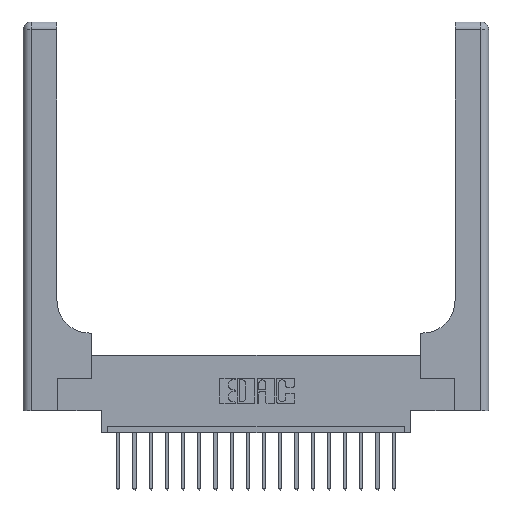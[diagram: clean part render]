
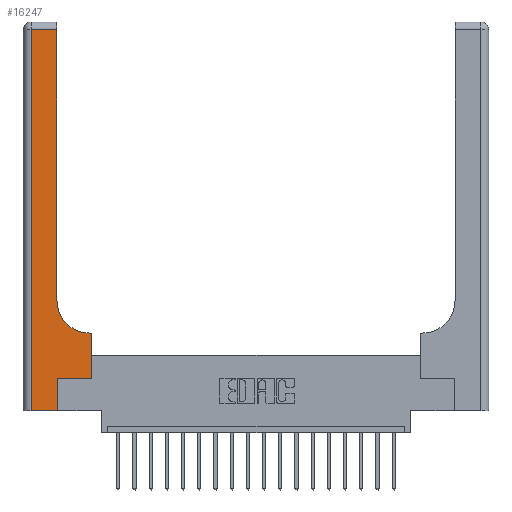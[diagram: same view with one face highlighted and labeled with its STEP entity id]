
A CAD part, top view. The second image highlights one B-rep face of the part: STEP entity #16247.
In plain terms, the highlighted planar face has unit normal (0, 0, 1).
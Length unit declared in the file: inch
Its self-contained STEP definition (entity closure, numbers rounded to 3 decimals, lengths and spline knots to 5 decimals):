
#728 = ORIENTED_EDGE ( 'NONE', *, *, #10570, .T. ) ;
#733 = FACE_OUTER_BOUND ( 'NONE', #19905, .T. ) ;
#1167 = CARTESIAN_POINT ( 'NONE',  ( 0.51, 0.6, 0.37 ) ) ;
#1189 = ORIENTED_EDGE ( 'NONE', *, *, #10052, .T. ) ;
#1239 = ORIENTED_EDGE ( 'NONE', *, *, #1798, .T. ) ;
#1676 = CARTESIAN_POINT ( 'NONE',  ( 0.51, 0.85, 0.37 ) ) ;
#1798 = EDGE_CURVE ( 'NONE', #15575, #12242, #14956, .T. ) ;
#2239 = CARTESIAN_POINT ( 'NONE',  ( 0.06, 0., 0.37 ) ) ;
#2600 = CARTESIAN_POINT ( 'NONE',  ( 0.26, 0.6, 0.37 ) ) ;
#2780 = ORIENTED_EDGE ( 'NONE', *, *, #17209, .T. ) ;
#3410 = DIRECTION ( 'NONE',  ( -1., 0., 0. ) ) ;
#4411 = DIRECTION ( 'NONE',  ( 1., 0., 0. ) ) ;
#4702 = CARTESIAN_POINT ( 'NONE',  ( 0.26, 0.85, 0.37 ) ) ;
#5264 = CARTESIAN_POINT ( 'NONE',  ( 0.06, 2.94, 0.37 ) ) ;
#5432 = VECTOR ( 'NONE', #12123, 39.37008 ) ;
#5564 = DIRECTION ( 'NONE',  ( -1., 0., 0. ) ) ;
#5778 = LINE ( 'NONE', #12019, #12979 ) ;
#5793 = LINE ( 'NONE', #12033, #10320 ) ;
#5887 = LINE ( 'NONE', #6471, #5432 ) ;
#5993 = EDGE_CURVE ( 'NONE', #12242, #11023, #7613, .T. ) ;
#6471 = CARTESIAN_POINT ( 'NONE',  ( 0.265, 0., 0.37 ) ) ;
#6580 = EDGE_CURVE ( 'NONE', #11023, #13014, #5793, .T. ) ;
#6800 = EDGE_CURVE ( 'NONE', #9918, #13828, #5887, .T. ) ;
#6950 = CARTESIAN_POINT ( 'NONE',  ( 0., 3., 0.37 ) ) ;
#7481 = CARTESIAN_POINT ( 'NONE',  ( 0.265, 0.25, 0.37 ) ) ;
#7613 = CIRCLE ( 'NONE', #16418, 0.25 ) ;
#7614 = VERTEX_POINT ( 'NONE', #2239 ) ;
#7651 = LINE ( 'NONE', #13686, #8323 ) ;
#7672 = VECTOR ( 'NONE', #3410, 39.37008 ) ;
#8037 = ORIENTED_EDGE ( 'NONE', *, *, #16269, .T. ) ;
#8323 = VECTOR ( 'NONE', #15114, 39.37008 ) ;
#8761 = VECTOR ( 'NONE', #4411, 39.37008 ) ;
#9447 = DIRECTION ( 'NONE',  ( 0., 0., -1. ) ) ;
#9918 = VERTEX_POINT ( 'NONE', #15132 ) ;
#10052 = EDGE_CURVE ( 'NONE', #13828, #17823, #15438, .T. ) ;
#10315 = CARTESIAN_POINT ( 'NONE',  ( 0.528, 0.25, 0.37 ) ) ;
#10320 = VECTOR ( 'NONE', #19772, 39.37008 ) ;
#10570 = EDGE_CURVE ( 'NONE', #7614, #9918, #13710, .T. ) ;
#11023 = VERTEX_POINT ( 'NONE', #4702 ) ;
#11766 = PLANE ( 'NONE',  #17117 ) ;
#12019 = CARTESIAN_POINT ( 'NONE',  ( 0.528, 0.25, 0.37 ) ) ;
#12033 = CARTESIAN_POINT ( 'NONE',  ( 0.26, 3., 0.37 ) ) ;
#12119 = CARTESIAN_POINT ( 'NONE',  ( 0.26, 2.94, 0.37 ) ) ;
#12123 = DIRECTION ( 'NONE',  ( 0., 1., 0. ) ) ;
#12242 = VERTEX_POINT ( 'NONE', #1167 ) ;
#12794 = DIRECTION ( 'NONE',  ( 1., 0., 0. ) ) ;
#12979 = VECTOR ( 'NONE', #18230, 39.37008 ) ;
#13007 = VECTOR ( 'NONE', #15348, 39.37008 ) ;
#13014 = VERTEX_POINT ( 'NONE', #12119 ) ;
#13178 = DIRECTION ( 'NONE',  ( 0., 0., -1. ) ) ;
#13226 = ORIENTED_EDGE ( 'NONE', *, *, #6800, .T. ) ;
#13445 = EDGE_CURVE ( 'NONE', #13014, #14250, #18615, .T. ) ;
#13686 = CARTESIAN_POINT ( 'NONE',  ( 0.06, 3., 0.37 ) ) ;
#13710 = LINE ( 'NONE', #17183, #13007 ) ;
#13828 = VERTEX_POINT ( 'NONE', #16317 ) ;
#14250 = VERTEX_POINT ( 'NONE', #5264 ) ;
#14956 = LINE ( 'NONE', #2600, #14977 ) ;
#14977 = VECTOR ( 'NONE', #5564, 39.37008 ) ;
#15114 = DIRECTION ( 'NONE',  ( 0., -1., 0. ) ) ;
#15132 = CARTESIAN_POINT ( 'NONE',  ( 0.265, 0., 0.37 ) ) ;
#15233 = ORIENTED_EDGE ( 'NONE', *, *, #5993, .T. ) ;
#15348 = DIRECTION ( 'NONE',  ( 1., 0., 0. ) ) ;
#15438 = LINE ( 'NONE', #7481, #8761 ) ;
#15575 = VERTEX_POINT ( 'NONE', #16994 ) ;
#16247 = ADVANCED_FACE ( 'NONE', ( #733 ), #11766, .F. ) ;
#16269 = EDGE_CURVE ( 'NONE', #14250, #7614, #7651, .T. ) ;
#16317 = CARTESIAN_POINT ( 'NONE',  ( 0.265, 0.25, 0.37 ) ) ;
#16418 = AXIS2_PLACEMENT_3D ( 'NONE', #1676, #9447, #12794 ) ;
#16441 = DIRECTION ( 'NONE',  ( -1., 0., 0. ) ) ;
#16994 = CARTESIAN_POINT ( 'NONE',  ( 0.528, 0.6, 0.37 ) ) ;
#17117 = AXIS2_PLACEMENT_3D ( 'NONE', #6950, #13178, #16441 ) ;
#17183 = CARTESIAN_POINT ( 'NONE',  ( 0., 0., 0.37 ) ) ;
#17209 = EDGE_CURVE ( 'NONE', #17823, #15575, #5778, .T. ) ;
#17823 = VERTEX_POINT ( 'NONE', #10315 ) ;
#18185 = ORIENTED_EDGE ( 'NONE', *, *, #6580, .T. ) ;
#18230 = DIRECTION ( 'NONE',  ( 0., 1., 0. ) ) ;
#18615 = LINE ( 'NONE', #19015, #7672 ) ;
#19015 = CARTESIAN_POINT ( 'NONE',  ( 0., 2.94, 0.37 ) ) ;
#19100 = ORIENTED_EDGE ( 'NONE', *, *, #13445, .T. ) ;
#19772 = DIRECTION ( 'NONE',  ( 0., 1., 0. ) ) ;
#19905 = EDGE_LOOP ( 'NONE', ( #18185, #19100, #8037, #728, #13226, #1189, #2780, #1239, #15233 ) ) ;
